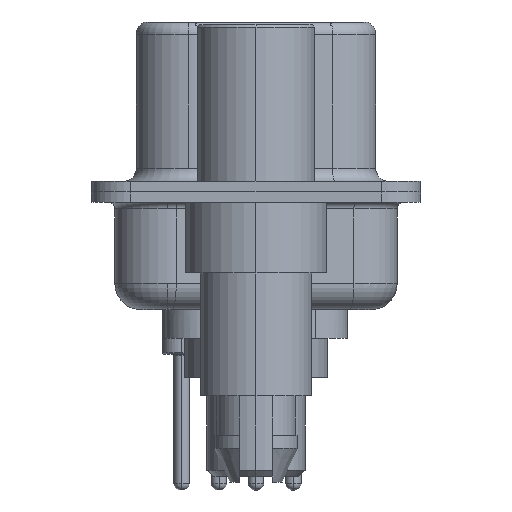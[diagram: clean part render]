
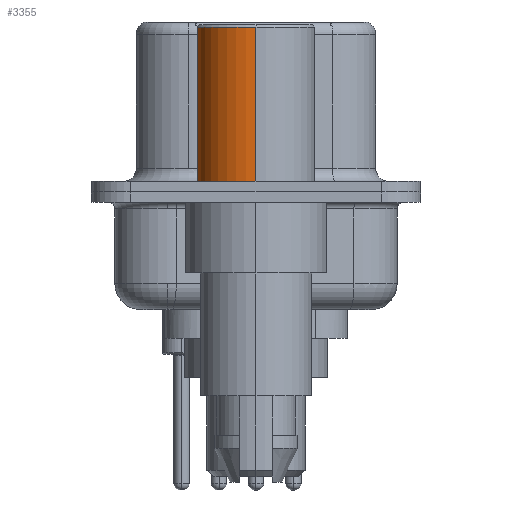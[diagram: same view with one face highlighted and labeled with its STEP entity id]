
A CAD part, left-side view. The second image highlights one B-rep face of the part: STEP entity #3355.
In plain terms, the highlighted cylindrical face has radius 2.25 mm (diameter 4.5 mm), a partial arc.
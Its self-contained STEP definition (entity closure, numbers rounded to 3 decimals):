
#2200 = EDGE_CURVE ( 'NONE', #9696, #20119, #22353, .T. ) ;
#2329 = AXIS2_PLACEMENT_3D ( 'NONE', #5638, #5607, #5559 ) ;
#2660 = EDGE_LOOP ( 'NONE', ( #8647, #22711, #14818, #3356 ) ) ;
#3089 = DIRECTION ( 'NONE',  ( 1., 0., 0. ) ) ;
#3355 = ADVANCED_FACE ( 'NONE', ( #13632 ), #22298, .T. ) ;
#3356 = ORIENTED_EDGE ( 'NONE', *, *, #2200, .F. ) ;
#4277 = CARTESIAN_POINT ( 'NONE',  ( 0., 0., 0.581 ) ) ;
#4524 = EDGE_CURVE ( 'NONE', #20119, #14148, #19869, .T. ) ;
#5559 = DIRECTION ( 'NONE',  ( 1., 0., 0. ) ) ;
#5607 = DIRECTION ( 'NONE',  ( 0., 0., 1. ) ) ;
#5638 = CARTESIAN_POINT ( 'NONE',  ( 0., 0., 0.4 ) ) ;
#7949 = DIRECTION ( 'NONE',  ( 0., 0., 1. ) ) ;
#8647 = ORIENTED_EDGE ( 'NONE', *, *, #9305, .T. ) ;
#9305 = EDGE_CURVE ( 'NONE', #9696, #20906, #13897, .T. ) ;
#9696 = VERTEX_POINT ( 'NONE', #19097 ) ;
#10047 = CARTESIAN_POINT ( 'NONE',  ( -2.25, 0., 0.4 ) ) ;
#10637 = AXIS2_PLACEMENT_3D ( 'NONE', #23832, #23825, #23751 ) ;
#11460 = LINE ( 'NONE', #11969, #16358 ) ;
#11969 = CARTESIAN_POINT ( 'NONE',  ( -2.25, 0., 0.581 ) ) ;
#13632 = FACE_OUTER_BOUND ( 'NONE', #2660, .T. ) ;
#13897 = CIRCLE ( 'NONE', #2329, 2.25 ) ;
#14148 = VERTEX_POINT ( 'NONE', #19679 ) ;
#14818 = ORIENTED_EDGE ( 'NONE', *, *, #4524, .F. ) ;
#15168 = CARTESIAN_POINT ( 'NONE',  ( 2.25, 0., 6.3 ) ) ;
#15789 = DIRECTION ( 'NONE',  ( 0., 0., 1. ) ) ;
#16358 = VECTOR ( 'NONE', #23023, 1000. ) ;
#17418 = VECTOR ( 'NONE', #7949, 1000. ) ;
#19097 = CARTESIAN_POINT ( 'NONE',  ( 2.25, 0., 0.4 ) ) ;
#19679 = CARTESIAN_POINT ( 'NONE',  ( -2.25, 0., 6.3 ) ) ;
#19869 = CIRCLE ( 'NONE', #10637, 2.25 ) ;
#20119 = VERTEX_POINT ( 'NONE', #15168 ) ;
#20306 = AXIS2_PLACEMENT_3D ( 'NONE', #4277, #15789, #3089 ) ;
#20906 = VERTEX_POINT ( 'NONE', #10047 ) ;
#20946 = EDGE_CURVE ( 'NONE', #20906, #14148, #11460, .T. ) ;
#21074 = CARTESIAN_POINT ( 'NONE',  ( 2.25, 0., 0.581 ) ) ;
#22298 = CYLINDRICAL_SURFACE ( 'NONE', #20306, 2.25 ) ;
#22353 = LINE ( 'NONE', #21074, #17418 ) ;
#22711 = ORIENTED_EDGE ( 'NONE', *, *, #20946, .T. ) ;
#23023 = DIRECTION ( 'NONE',  ( 0., 0., 1. ) ) ;
#23751 = DIRECTION ( 'NONE',  ( 1., 0., 0. ) ) ;
#23825 = DIRECTION ( 'NONE',  ( 0., 0., 1. ) ) ;
#23832 = CARTESIAN_POINT ( 'NONE',  ( 0., 0., 6.3 ) ) ;
